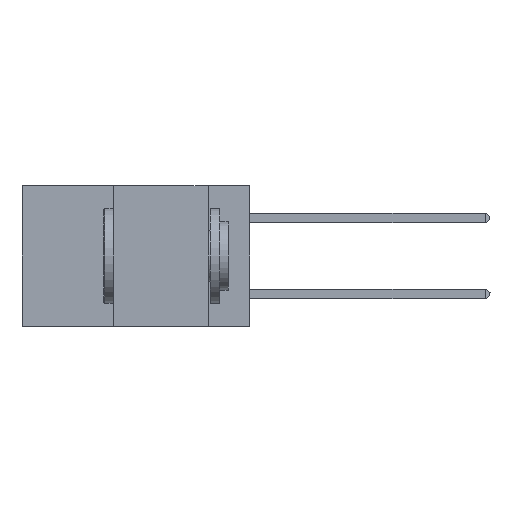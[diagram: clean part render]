
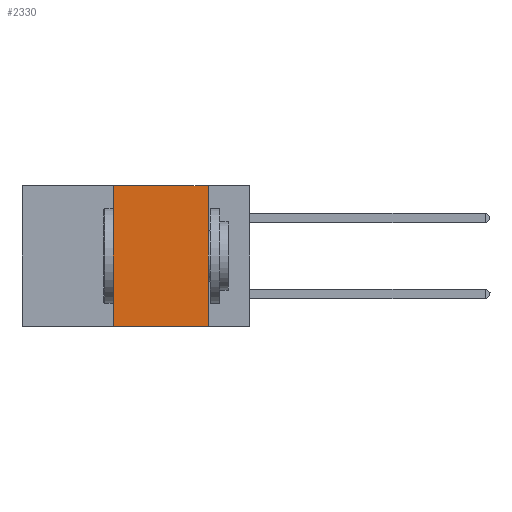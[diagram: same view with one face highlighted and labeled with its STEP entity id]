
A CAD part, left-side view. The second image highlights one B-rep face of the part: STEP entity #2330.
In plain terms, the highlighted planar face has unit normal (-1, 0, 0).
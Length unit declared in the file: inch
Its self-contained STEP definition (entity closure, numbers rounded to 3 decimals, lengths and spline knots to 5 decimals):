
#2330 = ADVANCED_FACE ( 'NONE', ( #23959 ), #23158, .F. ) ;
#4701 = EDGE_CURVE ( 'NONE', #36090, #13480, #17857, .T. ) ;
#4852 = ORIENTED_EDGE ( 'NONE', *, *, #4701, .T. ) ;
#4856 = AXIS2_PLACEMENT_3D ( 'NONE', #26583, #30058, #9385 ) ;
#6202 = DIRECTION ( 'NONE',  ( 0., -1., 0. ) ) ;
#6825 = EDGE_LOOP ( 'NONE', ( #28116, #10852, #20031, #4852 ) ) ;
#9385 = DIRECTION ( 'NONE',  ( 0., 0., -1. ) ) ;
#10852 = ORIENTED_EDGE ( 'NONE', *, *, #22892, .F. ) ;
#12817 = LINE ( 'NONE', #37182, #38189 ) ;
#13480 = VERTEX_POINT ( 'NONE', #41632 ) ;
#16888 = CARTESIAN_POINT ( 'NONE',  ( 0., 0.36, 0. ) ) ;
#17857 = LINE ( 'NONE', #20842, #35106 ) ;
#19234 = VERTEX_POINT ( 'NONE', #42049 ) ;
#20031 = ORIENTED_EDGE ( 'NONE', *, *, #27898, .F. ) ;
#20139 = CARTESIAN_POINT ( 'NONE',  ( 0., 0.11, 0. ) ) ;
#20842 = CARTESIAN_POINT ( 'NONE',  ( 0., 0.6, -0.37 ) ) ;
#22892 = EDGE_CURVE ( 'NONE', #19234, #36098, #12817, .T. ) ;
#23158 = PLANE ( 'NONE',  #4856 ) ;
#23467 = DIRECTION ( 'NONE',  ( 0., 0., -1. ) ) ;
#23959 = FACE_OUTER_BOUND ( 'NONE', #6825, .T. ) ;
#26583 = CARTESIAN_POINT ( 'NONE',  ( 0., 0.6, 0. ) ) ;
#26894 = CARTESIAN_POINT ( 'NONE',  ( 0., 0.11, 0. ) ) ;
#27811 = VECTOR ( 'NONE', #41004, 39.37008 ) ;
#27898 = EDGE_CURVE ( 'NONE', #36090, #19234, #43974, .T. ) ;
#28116 = ORIENTED_EDGE ( 'NONE', *, *, #29940, .F. ) ;
#29940 = EDGE_CURVE ( 'NONE', #36098, #13480, #34085, .T. ) ;
#30058 = DIRECTION ( 'NONE',  ( 1., 0., 0. ) ) ;
#34085 = LINE ( 'NONE', #26894, #42173 ) ;
#35106 = VECTOR ( 'NONE', #41457, 39.37008 ) ;
#36090 = VERTEX_POINT ( 'NONE', #44232 ) ;
#36098 = VERTEX_POINT ( 'NONE', #20139 ) ;
#37182 = CARTESIAN_POINT ( 'NONE',  ( 0., 0.6, 0. ) ) ;
#38189 = VECTOR ( 'NONE', #6202, 39.37008 ) ;
#41004 = DIRECTION ( 'NONE',  ( 0., 0., 1. ) ) ;
#41457 = DIRECTION ( 'NONE',  ( 0., -1., 0. ) ) ;
#41632 = CARTESIAN_POINT ( 'NONE',  ( 0., 0.11, -0.37 ) ) ;
#42049 = CARTESIAN_POINT ( 'NONE',  ( 0., 0.36, 0. ) ) ;
#42173 = VECTOR ( 'NONE', #23467, 39.37008 ) ;
#43974 = LINE ( 'NONE', #16888, #27811 ) ;
#44232 = CARTESIAN_POINT ( 'NONE',  ( 0., 0.36, -0.37 ) ) ;
